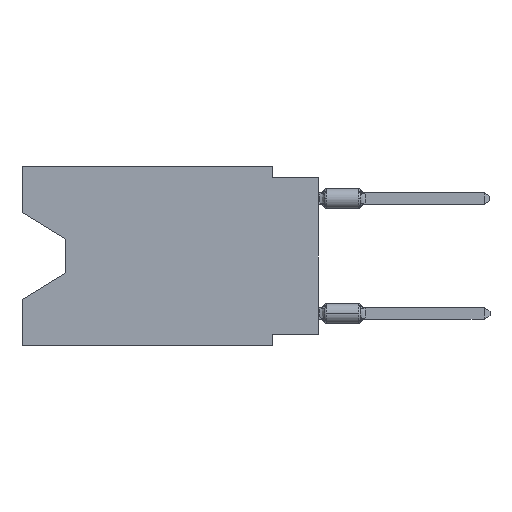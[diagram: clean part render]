
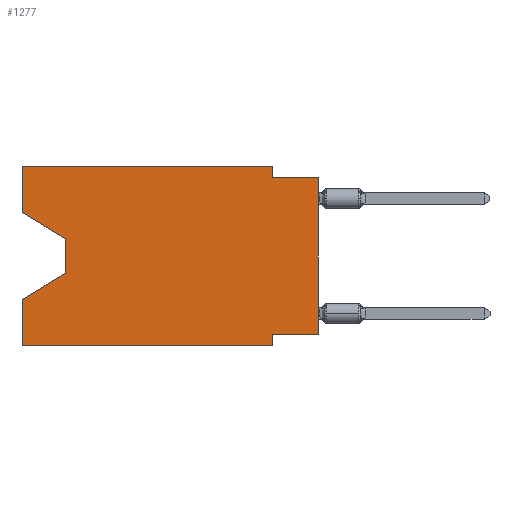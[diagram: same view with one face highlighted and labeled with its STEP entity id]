
A CAD part, left-side view. The second image highlights one B-rep face of the part: STEP entity #1277.
In plain terms, the highlighted planar face has unit normal (-1, 0, 0).
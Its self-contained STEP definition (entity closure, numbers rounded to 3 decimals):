
#233 = CARTESIAN_POINT ( 'NONE',  ( 0., 0., -0.635 ) ) ;
#368 = LINE ( 'NONE', #16141, #5460 ) ;
#603 = CARTESIAN_POINT ( 'NONE',  ( 0., 13.97, -5.893 ) ) ;
#632 = ORIENTED_EDGE ( 'NONE', *, *, #9197, .F. ) ;
#815 = DIRECTION ( 'NONE',  ( 0., -1., 0. ) ) ;
#1277 = ADVANCED_FACE ( 'NONE', ( #18855 ), #11372, .F. ) ;
#1430 = VERTEX_POINT ( 'NONE', #15005 ) ;
#1443 = DIRECTION ( 'NONE',  ( 0., 0., -1. ) ) ;
#1488 = ORIENTED_EDGE ( 'NONE', *, *, #17504, .F. ) ;
#1721 = VERTEX_POINT ( 'NONE', #2744 ) ;
#1886 = CARTESIAN_POINT ( 'NONE',  ( 0., 2.54, 0. ) ) ;
#2288 = CARTESIAN_POINT ( 'NONE',  ( 0., 0., -0.635 ) ) ;
#2425 = VERTEX_POINT ( 'NONE', #603 ) ;
#2642 = EDGE_CURVE ( 'NONE', #18194, #19081, #9200, .T. ) ;
#2647 = VECTOR ( 'NONE', #6948, 1000. ) ;
#2727 = VECTOR ( 'NONE', #17924, 1000. ) ;
#2744 = CARTESIAN_POINT ( 'NONE',  ( 0., 13.97, -4.013 ) ) ;
#2818 = EDGE_CURVE ( 'NONE', #3534, #1721, #14428, .T. ) ;
#3149 = VECTOR ( 'NONE', #4588, 1000. ) ;
#3400 = DIRECTION ( 'NONE',  ( 1., 0., 0. ) ) ;
#3523 = DIRECTION ( 'NONE',  ( 0., -1., 0. ) ) ;
#3534 = VERTEX_POINT ( 'NONE', #6981 ) ;
#3688 = VECTOR ( 'NONE', #14210, 1000. ) ;
#4161 = CARTESIAN_POINT ( 'NONE',  ( 0., 16.383, -7.36 ) ) ;
#4392 = CARTESIAN_POINT ( 'NONE',  ( 0., 16.383, -9.906 ) ) ;
#4588 = DIRECTION ( 'NONE',  ( 0., -1., 0. ) ) ;
#4610 = VECTOR ( 'NONE', #1443, 1000. ) ;
#4666 = EDGE_CURVE ( 'NONE', #15478, #15032, #14506, .T. ) ;
#5235 = LINE ( 'NONE', #2288, #12775 ) ;
#5273 = CARTESIAN_POINT ( 'NONE',  ( 0., 16.383, 0. ) ) ;
#5449 = VERTEX_POINT ( 'NONE', #5273 ) ;
#5460 = VECTOR ( 'NONE', #14609, 1000. ) ;
#5802 = EDGE_CURVE ( 'NONE', #2425, #15032, #18571, .T. ) ;
#6022 = ORIENTED_EDGE ( 'NONE', *, *, #4666, .F. ) ;
#6252 = VECTOR ( 'NONE', #12101, 1000. ) ;
#6385 = ORIENTED_EDGE ( 'NONE', *, *, #11513, .F. ) ;
#6948 = DIRECTION ( 'NONE',  ( 0., 0., 1. ) ) ;
#6981 = CARTESIAN_POINT ( 'NONE',  ( 0., 16.383, -2.546 ) ) ;
#7634 = CARTESIAN_POINT ( 'NONE',  ( 0., 2.54, -9.906 ) ) ;
#7657 = VERTEX_POINT ( 'NONE', #8730 ) ;
#7773 = DIRECTION ( 'NONE',  ( 0., 0., -1. ) ) ;
#8035 = ORIENTED_EDGE ( 'NONE', *, *, #2642, .F. ) ;
#8506 = LINE ( 'NONE', #14656, #10888 ) ;
#8639 = ORIENTED_EDGE ( 'NONE', *, *, #16921, .F. ) ;
#8730 = CARTESIAN_POINT ( 'NONE',  ( 0., 2.54, -9.906 ) ) ;
#8843 = VECTOR ( 'NONE', #17367, 1000. ) ;
#9151 = CARTESIAN_POINT ( 'NONE',  ( 0., 0., -9.271 ) ) ;
#9197 = EDGE_CURVE ( 'NONE', #5449, #1430, #8506, .T. ) ;
#9200 = LINE ( 'NONE', #19896, #6252 ) ;
#9875 = DIRECTION ( 'NONE',  ( 0., 0., -1. ) ) ;
#9897 = LINE ( 'NONE', #11674, #2647 ) ;
#9916 = CARTESIAN_POINT ( 'NONE',  ( 0., 2.54, -0.635 ) ) ;
#10429 = AXIS2_PLACEMENT_3D ( 'NONE', #17537, #3400, #9875 ) ;
#10565 = LINE ( 'NONE', #4392, #3149 ) ;
#10631 = ORIENTED_EDGE ( 'NONE', *, *, #18983, .F. ) ;
#10888 = VECTOR ( 'NONE', #815, 1000. ) ;
#10974 = EDGE_CURVE ( 'NONE', #18194, #11747, #9897, .T. ) ;
#10990 = CARTESIAN_POINT ( 'NONE',  ( 0., 13.97, -5.893 ) ) ;
#11180 = CARTESIAN_POINT ( 'NONE',  ( 0., 16.383, 0. ) ) ;
#11372 = PLANE ( 'NONE',  #10429 ) ;
#11513 = EDGE_CURVE ( 'NONE', #19081, #7657, #15293, .T. ) ;
#11674 = CARTESIAN_POINT ( 'NONE',  ( 0., 0., 0. ) ) ;
#11697 = CARTESIAN_POINT ( 'NONE',  ( 0., 16.383, -9.906 ) ) ;
#11739 = ORIENTED_EDGE ( 'NONE', *, *, #5802, .T. ) ;
#11747 = VERTEX_POINT ( 'NONE', #233 ) ;
#12101 = DIRECTION ( 'NONE',  ( 0., 1., 0. ) ) ;
#12771 = VECTOR ( 'NONE', #7773, 1000. ) ;
#12775 = VECTOR ( 'NONE', #3523, 1000. ) ;
#13362 = LINE ( 'NONE', #15099, #2727 ) ;
#13570 = ORIENTED_EDGE ( 'NONE', *, *, #13989, .T. ) ;
#13989 = EDGE_CURVE ( 'NONE', #15478, #7657, #10565, .T. ) ;
#14210 = DIRECTION ( 'NONE',  ( 0., 0.855, -0.519 ) ) ;
#14428 = LINE ( 'NONE', #16054, #8843 ) ;
#14506 = LINE ( 'NONE', #11180, #17602 ) ;
#14609 = DIRECTION ( 'NONE',  ( 0., 0., -1. ) ) ;
#14656 = CARTESIAN_POINT ( 'NONE',  ( 0., 16.383, 0. ) ) ;
#15005 = CARTESIAN_POINT ( 'NONE',  ( 0., 2.54, 0. ) ) ;
#15032 = VERTEX_POINT ( 'NONE', #4161 ) ;
#15099 = CARTESIAN_POINT ( 'NONE',  ( 0., 16.383, 0. ) ) ;
#15293 = LINE ( 'NONE', #7634, #4610 ) ;
#15386 = VERTEX_POINT ( 'NONE', #9916 ) ;
#15445 = LINE ( 'NONE', #1886, #12771 ) ;
#15478 = VERTEX_POINT ( 'NONE', #11697 ) ;
#15747 = EDGE_CURVE ( 'NONE', #1721, #2425, #368, .T. ) ;
#15802 = ORIENTED_EDGE ( 'NONE', *, *, #2818, .T. ) ;
#16054 = CARTESIAN_POINT ( 'NONE',  ( 0., 16.383, -2.546 ) ) ;
#16141 = CARTESIAN_POINT ( 'NONE',  ( 0., 13.97, -4.013 ) ) ;
#16921 = EDGE_CURVE ( 'NONE', #15386, #11747, #5235, .T. ) ;
#17367 = DIRECTION ( 'NONE',  ( 0., -0.855, -0.519 ) ) ;
#17504 = EDGE_CURVE ( 'NONE', #3534, #5449, #13362, .T. ) ;
#17537 = CARTESIAN_POINT ( 'NONE',  ( 0., 16.383, 0. ) ) ;
#17602 = VECTOR ( 'NONE', #17737, 1000. ) ;
#17657 = ORIENTED_EDGE ( 'NONE', *, *, #10974, .T. ) ;
#17737 = DIRECTION ( 'NONE',  ( 0., 0., 1. ) ) ;
#17856 = ORIENTED_EDGE ( 'NONE', *, *, #15747, .T. ) ;
#17924 = DIRECTION ( 'NONE',  ( 0., 0., 1. ) ) ;
#18194 = VERTEX_POINT ( 'NONE', #9151 ) ;
#18571 = LINE ( 'NONE', #10990, #3688 ) ;
#18673 = CARTESIAN_POINT ( 'NONE',  ( 0., 2.54, -9.271 ) ) ;
#18855 = FACE_OUTER_BOUND ( 'NONE', #19545, .T. ) ;
#18983 = EDGE_CURVE ( 'NONE', #1430, #15386, #15445, .T. ) ;
#19081 = VERTEX_POINT ( 'NONE', #18673 ) ;
#19545 = EDGE_LOOP ( 'NONE', ( #15802, #17856, #11739, #6022, #13570, #6385, #8035, #17657, #8639, #10631, #632, #1488 ) ) ;
#19896 = CARTESIAN_POINT ( 'NONE',  ( 0., 0., -9.271 ) ) ;
